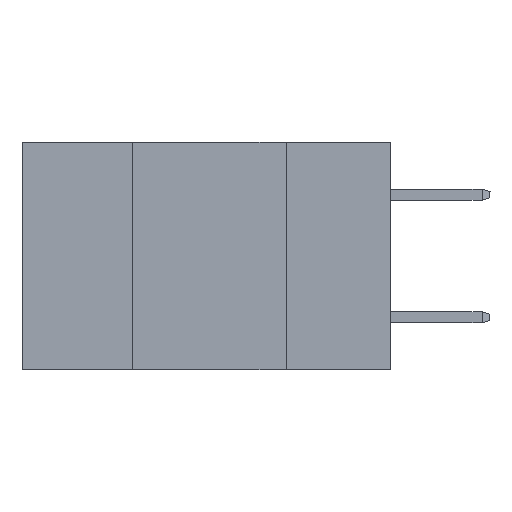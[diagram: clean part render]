
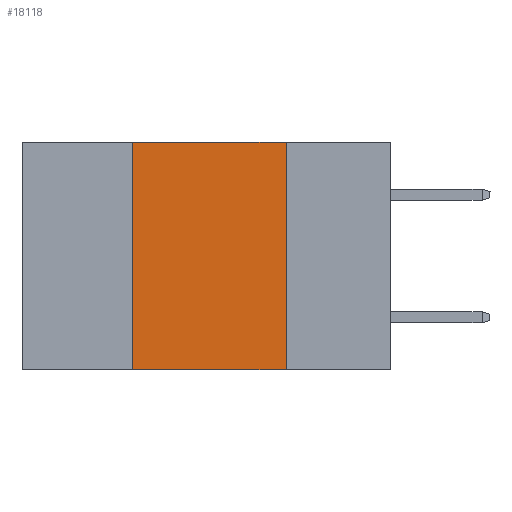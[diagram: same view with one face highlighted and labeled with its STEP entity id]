
A CAD part, left-side view. The second image highlights one B-rep face of the part: STEP entity #18118.
In plain terms, the highlighted planar face has unit normal (-1, 0, 0).
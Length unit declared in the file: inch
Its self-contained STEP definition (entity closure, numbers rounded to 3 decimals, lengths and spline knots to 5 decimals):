
#467 = CARTESIAN_POINT ( 'NONE',  ( 0., 0.17, -0.37 ) ) ;
#1044 = EDGE_LOOP ( 'NONE', ( #7301, #26593, #19486, #23660 ) ) ;
#1228 = VERTEX_POINT ( 'NONE', #22627 ) ;
#2073 = VECTOR ( 'NONE', #12181, 39.37008 ) ;
#3193 = PLANE ( 'NONE',  #26170 ) ;
#6438 = CARTESIAN_POINT ( 'NONE',  ( 0., 0.6, -0.37 ) ) ;
#7301 = ORIENTED_EDGE ( 'NONE', *, *, #12175, .F. ) ;
#9044 = CARTESIAN_POINT ( 'NONE',  ( 0., 0.42, -0.37 ) ) ;
#9973 = LINE ( 'NONE', #6438, #35195 ) ;
#11635 = CARTESIAN_POINT ( 'NONE',  ( 0., 0.17, 0. ) ) ;
#12175 = EDGE_CURVE ( 'NONE', #1228, #14151, #31936, .T. ) ;
#12181 = DIRECTION ( 'NONE',  ( 0., 0., -1. ) ) ;
#14151 = VERTEX_POINT ( 'NONE', #467 ) ;
#14778 = VECTOR ( 'NONE', #36327, 39.37008 ) ;
#15950 = VERTEX_POINT ( 'NONE', #9044 ) ;
#17097 = EDGE_CURVE ( 'NONE', #27052, #1228, #33143, .T. ) ;
#18071 = CARTESIAN_POINT ( 'NONE',  ( 0., 0.42, 0. ) ) ;
#18118 = ADVANCED_FACE ( 'NONE', ( #23570 ), #3193, .F. ) ;
#18303 = DIRECTION ( 'NONE',  ( 0., 0., -1. ) ) ;
#19486 = ORIENTED_EDGE ( 'NONE', *, *, #36577, .F. ) ;
#20667 = DIRECTION ( 'NONE',  ( 0., -1., 0. ) ) ;
#21133 = DIRECTION ( 'NONE',  ( 1., 0., 0. ) ) ;
#22627 = CARTESIAN_POINT ( 'NONE',  ( 0., 0.17, 0. ) ) ;
#23570 = FACE_OUTER_BOUND ( 'NONE', #1044, .T. ) ;
#23660 = ORIENTED_EDGE ( 'NONE', *, *, #32638, .T. ) ;
#26170 = AXIS2_PLACEMENT_3D ( 'NONE', #35255, #21133, #18303 ) ;
#26593 = ORIENTED_EDGE ( 'NONE', *, *, #17097, .F. ) ;
#26994 = VECTOR ( 'NONE', #29433, 39.37008 ) ;
#27052 = VERTEX_POINT ( 'NONE', #36626 ) ;
#28324 = CARTESIAN_POINT ( 'NONE',  ( 0., 0.6, 0. ) ) ;
#29433 = DIRECTION ( 'NONE',  ( 0., 0., 1. ) ) ;
#31936 = LINE ( 'NONE', #11635, #2073 ) ;
#32221 = LINE ( 'NONE', #18071, #26994 ) ;
#32638 = EDGE_CURVE ( 'NONE', #15950, #14151, #9973, .T. ) ;
#33143 = LINE ( 'NONE', #28324, #14778 ) ;
#35195 = VECTOR ( 'NONE', #20667, 39.37008 ) ;
#35255 = CARTESIAN_POINT ( 'NONE',  ( 0., 0.6, 0. ) ) ;
#36327 = DIRECTION ( 'NONE',  ( 0., -1., 0. ) ) ;
#36577 = EDGE_CURVE ( 'NONE', #15950, #27052, #32221, .T. ) ;
#36626 = CARTESIAN_POINT ( 'NONE',  ( 0., 0.42, 0. ) ) ;
